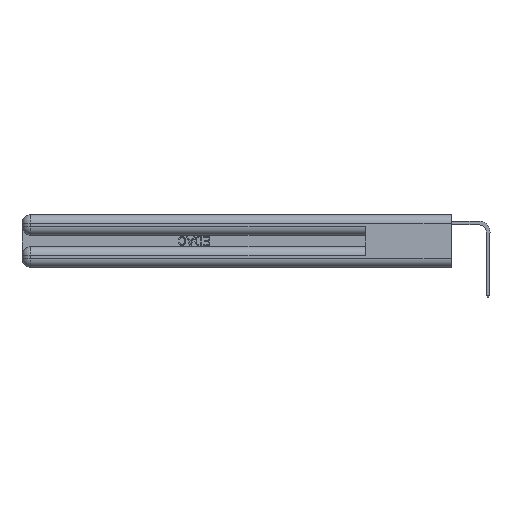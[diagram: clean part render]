
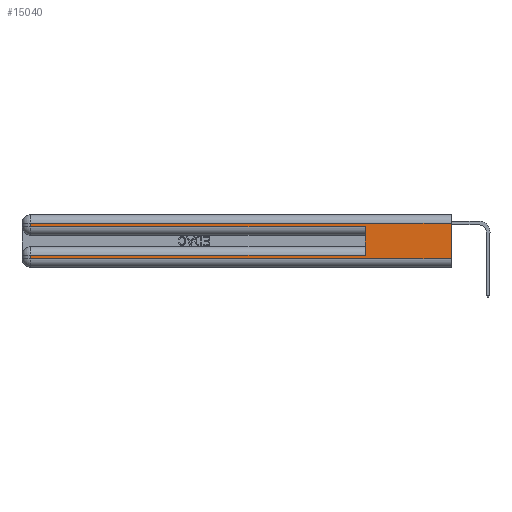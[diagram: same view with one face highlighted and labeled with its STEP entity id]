
A CAD part, left-side view. The second image highlights one B-rep face of the part: STEP entity #15040.
In plain terms, the highlighted planar face has unit normal (-1, 0, 0).
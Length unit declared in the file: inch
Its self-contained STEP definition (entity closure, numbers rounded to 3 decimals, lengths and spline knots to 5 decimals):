
#214 = DIRECTION ( 'NONE',  ( 0., 1., 0. ) ) ;
#310 = CARTESIAN_POINT ( 'NONE',  ( 0., 2.94, 0.37 ) ) ;
#325 = EDGE_LOOP ( 'NONE', ( #24234, #19061, #27064, #27147, #23865, #18510, #18591, #18153 ) ) ;
#431 = EDGE_CURVE ( 'NONE', #5402, #24487, #21659, .T. ) ;
#606 = VECTOR ( 'NONE', #29248, 39.37008 ) ;
#969 = FACE_OUTER_BOUND ( 'NONE', #325, .T. ) ;
#1658 = VERTEX_POINT ( 'NONE', #21128 ) ;
#2002 = EDGE_CURVE ( 'NONE', #24487, #22237, #13686, .T. ) ;
#2655 = DIRECTION ( 'NONE',  ( 0., 0., -1. ) ) ;
#2789 = LINE ( 'NONE', #4120, #20501 ) ;
#3255 = VECTOR ( 'NONE', #20892, 39.37008 ) ;
#3560 = EDGE_CURVE ( 'NONE', #22237, #16343, #22921, .T. ) ;
#4120 = CARTESIAN_POINT ( 'NONE',  ( 0., 0.6, 0.145 ) ) ;
#5402 = VERTEX_POINT ( 'NONE', #20996 ) ;
#5788 = VECTOR ( 'NONE', #2655, 39.37008 ) ;
#6415 = DIRECTION ( 'NONE',  ( 0., 0., 1. ) ) ;
#7898 = CARTESIAN_POINT ( 'NONE',  ( 0., 2.94, 0.085 ) ) ;
#8845 = DIRECTION ( 'NONE',  ( 0., -1., 0. ) ) ;
#8931 = LINE ( 'NONE', #16426, #14393 ) ;
#9045 = PLANE ( 'NONE',  #21395 ) ;
#9385 = CARTESIAN_POINT ( 'NONE',  ( 0., 0., 0.06 ) ) ;
#9666 = VERTEX_POINT ( 'NONE', #27876 ) ;
#10310 = EDGE_CURVE ( 'NONE', #1658, #20226, #8931, .T. ) ;
#10495 = VECTOR ( 'NONE', #24957, 39.37008 ) ;
#10838 = CARTESIAN_POINT ( 'NONE',  ( 0., 2.94, 0.37 ) ) ;
#10948 = LINE ( 'NONE', #24956, #23183 ) ;
#11230 = VERTEX_POINT ( 'NONE', #22328 ) ;
#11400 = DIRECTION ( 'NONE',  ( 1., 0., 0. ) ) ;
#11625 = CARTESIAN_POINT ( 'NONE',  ( 0., 2.94, 0.06 ) ) ;
#11951 = LINE ( 'NONE', #310, #5788 ) ;
#13686 = LINE ( 'NONE', #10838, #606 ) ;
#14393 = VECTOR ( 'NONE', #214, 39.37008 ) ;
#14881 = CARTESIAN_POINT ( 'NONE',  ( 0., 2.94, 0.31 ) ) ;
#15040 = ADVANCED_FACE ( 'NONE', ( #969 ), #9045, .F. ) ;
#16343 = VERTEX_POINT ( 'NONE', #9385 ) ;
#16426 = CARTESIAN_POINT ( 'NONE',  ( 0., 0., 0.31 ) ) ;
#16826 = VECTOR ( 'NONE', #29715, 39.37008 ) ;
#18153 = ORIENTED_EDGE ( 'NONE', *, *, #3560, .T. ) ;
#18510 = ORIENTED_EDGE ( 'NONE', *, *, #431, .T. ) ;
#18591 = ORIENTED_EDGE ( 'NONE', *, *, #2002, .T. ) ;
#18606 = CARTESIAN_POINT ( 'NONE',  ( 0., 0., 0.085 ) ) ;
#19061 = ORIENTED_EDGE ( 'NONE', *, *, #10310, .T. ) ;
#19604 = EDGE_CURVE ( 'NONE', #1658, #16343, #29601, .T. ) ;
#20226 = VERTEX_POINT ( 'NONE', #14881 ) ;
#20501 = VECTOR ( 'NONE', #6415, 39.37008 ) ;
#20892 = DIRECTION ( 'NONE',  ( 0., 1., 0. ) ) ;
#20996 = CARTESIAN_POINT ( 'NONE',  ( 0., 0.6, 0.085 ) ) ;
#21128 = CARTESIAN_POINT ( 'NONE',  ( 0., 0., 0.31 ) ) ;
#21141 = EDGE_CURVE ( 'NONE', #9666, #11230, #10948, .T. ) ;
#21395 = AXIS2_PLACEMENT_3D ( 'NONE', #25159, #11400, #27470 ) ;
#21659 = LINE ( 'NONE', #18606, #3255 ) ;
#22237 = VERTEX_POINT ( 'NONE', #11625 ) ;
#22328 = CARTESIAN_POINT ( 'NONE',  ( 0., 0.6, 0.285 ) ) ;
#22663 = CARTESIAN_POINT ( 'NONE',  ( 0., 0., 0.37 ) ) ;
#22685 = EDGE_CURVE ( 'NONE', #20226, #9666, #11951, .T. ) ;
#22785 = CARTESIAN_POINT ( 'NONE',  ( 0., 0., 0.06 ) ) ;
#22921 = LINE ( 'NONE', #22785, #16826 ) ;
#23183 = VECTOR ( 'NONE', #8845, 39.37008 ) ;
#23865 = ORIENTED_EDGE ( 'NONE', *, *, #24207, .F. ) ;
#24207 = EDGE_CURVE ( 'NONE', #5402, #11230, #2789, .T. ) ;
#24234 = ORIENTED_EDGE ( 'NONE', *, *, #19604, .F. ) ;
#24487 = VERTEX_POINT ( 'NONE', #7898 ) ;
#24956 = CARTESIAN_POINT ( 'NONE',  ( 0., 0., 0.285 ) ) ;
#24957 = DIRECTION ( 'NONE',  ( 0., 0., -1. ) ) ;
#25159 = CARTESIAN_POINT ( 'NONE',  ( 0., 0., 0.37 ) ) ;
#27064 = ORIENTED_EDGE ( 'NONE', *, *, #22685, .T. ) ;
#27147 = ORIENTED_EDGE ( 'NONE', *, *, #21141, .T. ) ;
#27470 = DIRECTION ( 'NONE',  ( 0., 0., -1. ) ) ;
#27876 = CARTESIAN_POINT ( 'NONE',  ( 0., 2.94, 0.285 ) ) ;
#29248 = DIRECTION ( 'NONE',  ( 0., 0., -1. ) ) ;
#29601 = LINE ( 'NONE', #22663, #10495 ) ;
#29715 = DIRECTION ( 'NONE',  ( 0., -1., 0. ) ) ;
